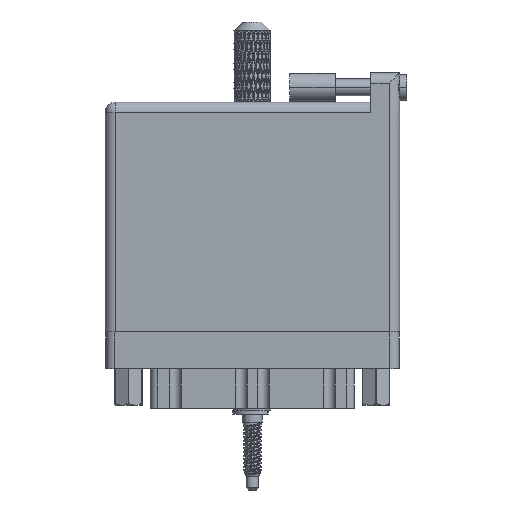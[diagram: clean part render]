
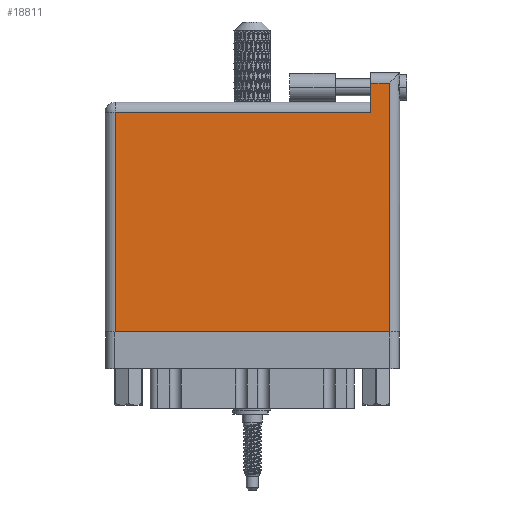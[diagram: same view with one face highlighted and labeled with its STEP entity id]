
A CAD part, front view. The second image highlights one B-rep face of the part: STEP entity #18811.
In plain terms, the highlighted face is planar.
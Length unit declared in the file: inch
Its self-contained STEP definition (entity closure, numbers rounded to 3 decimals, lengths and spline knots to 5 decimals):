
#2767 = LINE ( 'NONE', #38162, #46772 ) ;
#5666 = CARTESIAN_POINT ( 'NONE',  ( 0.07, 1.496, 0. ) ) ;
#5832 = ORIENTED_EDGE ( 'NONE', *, *, #6330, .T. ) ;
#6330 = EDGE_CURVE ( 'NONE', #75349, #44026, #55034, .T. ) ;
#6361 = ORIENTED_EDGE ( 'NONE', *, *, #60029, .T. ) ;
#6650 = VERTEX_POINT ( 'NONE', #64606 ) ;
#7222 = DIRECTION ( 'NONE',  ( 0., 0., -1. ) ) ;
#7769 = FACE_OUTER_BOUND ( 'NONE', #23915, .T. ) ;
#7980 = VERTEX_POINT ( 'NONE', #72459 ) ;
#18811 = ADVANCED_FACE ( 'NONE', ( #7769 ), #59177, .F. ) ;
#19559 = VECTOR ( 'NONE', #75687, 39.37008 ) ;
#20758 = LINE ( 'NONE', #98952, #34642 ) ;
#23287 = CARTESIAN_POINT ( 'NONE',  ( 0., 1.566, 0. ) ) ;
#23633 = CARTESIAN_POINT ( 'NONE',  ( 1.938, 0., 0. ) ) ;
#23915 = EDGE_LOOP ( 'NONE', ( #5832, #28750, #6361, #77481, #100527, #44261 ) ) ;
#24112 = CARTESIAN_POINT ( 'NONE',  ( 0.07, 0., 0. ) ) ;
#24224 = EDGE_CURVE ( 'NONE', #44026, #108361, #75166, .T. ) ;
#28750 = ORIENTED_EDGE ( 'NONE', *, *, #24224, .T. ) ;
#29653 = AXIS2_PLACEMENT_3D ( 'NONE', #23287, #7222, #40900 ) ;
#30473 = CARTESIAN_POINT ( 'NONE',  ( 0., 0., 0. ) ) ;
#34642 = VECTOR ( 'NONE', #55522, 39.37008 ) ;
#38162 = CARTESIAN_POINT ( 'NONE',  ( 0.07, 0., 0. ) ) ;
#40900 = DIRECTION ( 'NONE',  ( -1., 0., 0. ) ) ;
#44026 = VERTEX_POINT ( 'NONE', #23633 ) ;
#44261 = ORIENTED_EDGE ( 'NONE', *, *, #109153, .T. ) ;
#46375 = VECTOR ( 'NONE', #99009, 39.37008 ) ;
#46444 = DIRECTION ( 'NONE',  ( 1., 0., 0. ) ) ;
#46772 = VECTOR ( 'NONE', #81578, 39.37008 ) ;
#54179 = EDGE_CURVE ( 'NONE', #6650, #7980, #81285, .T. ) ;
#55034 = LINE ( 'NONE', #30473, #80123 ) ;
#55522 = DIRECTION ( 'NONE',  ( -1., 0., 0. ) ) ;
#59177 = PLANE ( 'NONE',  #29653 ) ;
#59929 = CARTESIAN_POINT ( 'NONE',  ( 1.938, 1.696, 0. ) ) ;
#60029 = EDGE_CURVE ( 'NONE', #108361, #6650, #83709, .T. ) ;
#64606 = CARTESIAN_POINT ( 'NONE',  ( 1.811, 1.696, 0. ) ) ;
#72459 = CARTESIAN_POINT ( 'NONE',  ( 1.811, 1.496, 0. ) ) ;
#75166 = LINE ( 'NONE', #92909, #78507 ) ;
#75349 = VERTEX_POINT ( 'NONE', #24112 ) ;
#75687 = DIRECTION ( 'NONE',  ( -1., 0., 0. ) ) ;
#77481 = ORIENTED_EDGE ( 'NONE', *, *, #54179, .T. ) ;
#78507 = VECTOR ( 'NONE', #110062, 39.37008 ) ;
#80123 = VECTOR ( 'NONE', #46444, 39.37008 ) ;
#81285 = LINE ( 'NONE', #96750, #46375 ) ;
#81578 = DIRECTION ( 'NONE',  ( 0., -1., 0. ) ) ;
#83709 = LINE ( 'NONE', #93431, #19559 ) ;
#92909 = CARTESIAN_POINT ( 'NONE',  ( 1.938, 1.766, 0. ) ) ;
#93431 = CARTESIAN_POINT ( 'NONE',  ( 0., 1.696, 0. ) ) ;
#96750 = CARTESIAN_POINT ( 'NONE',  ( 1.811, 1.766, 0. ) ) ;
#98952 = CARTESIAN_POINT ( 'NONE',  ( 0., 1.496, 0. ) ) ;
#99009 = DIRECTION ( 'NONE',  ( 0., -1., 0. ) ) ;
#99830 = VERTEX_POINT ( 'NONE', #5666 ) ;
#100527 = ORIENTED_EDGE ( 'NONE', *, *, #105202, .T. ) ;
#105202 = EDGE_CURVE ( 'NONE', #7980, #99830, #20758, .T. ) ;
#108361 = VERTEX_POINT ( 'NONE', #59929 ) ;
#109153 = EDGE_CURVE ( 'NONE', #99830, #75349, #2767, .T. ) ;
#110062 = DIRECTION ( 'NONE',  ( 0., 1., 0. ) ) ;
